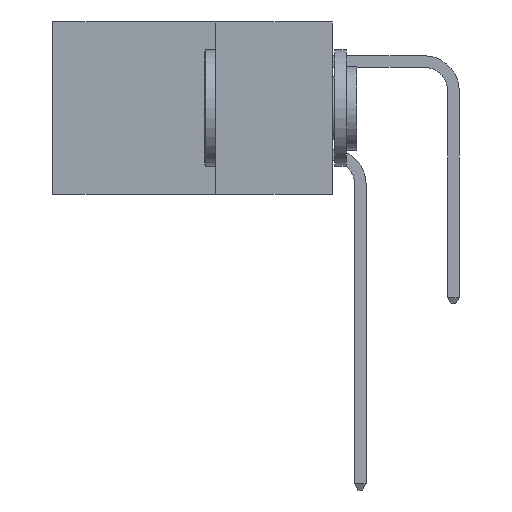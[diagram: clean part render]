
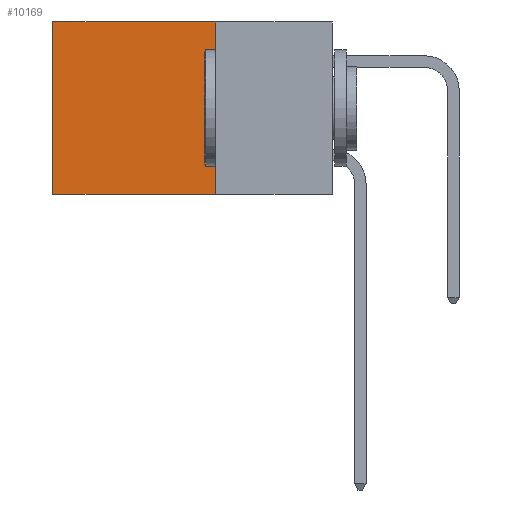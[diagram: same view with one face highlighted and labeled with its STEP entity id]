
A CAD part, left-side view. The second image highlights one B-rep face of the part: STEP entity #10169.
In plain terms, the highlighted planar face has unit normal (-1, 0, 0).
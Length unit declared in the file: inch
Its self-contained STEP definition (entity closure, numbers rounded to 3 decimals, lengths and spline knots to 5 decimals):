
#74 = LINE ( 'NONE', #7665, #5680 ) ;
#1587 = VECTOR ( 'NONE', #6917, 39.37008 ) ;
#1938 = VECTOR ( 'NONE', #3022, 39.37008 ) ;
#3015 = EDGE_LOOP ( 'NONE', ( #4439, #4606, #4668, #4705 ) ) ;
#3022 = DIRECTION ( 'NONE',  ( 0., 1., 0. ) ) ;
#3289 = VERTEX_POINT ( 'NONE', #12738 ) ;
#3512 = DIRECTION ( 'NONE',  ( 0., 0., -1. ) ) ;
#3734 = EDGE_CURVE ( 'NONE', #8182, #3289, #6736, .T. ) ;
#3924 = VECTOR ( 'NONE', #13265, 39.37008 ) ;
#4439 = ORIENTED_EDGE ( 'NONE', *, *, #6922, .T. ) ;
#4606 = ORIENTED_EDGE ( 'NONE', *, *, #10171, .F. ) ;
#4668 = ORIENTED_EDGE ( 'NONE', *, *, #6403, .F. ) ;
#4705 = ORIENTED_EDGE ( 'NONE', *, *, #3734, .T. ) ;
#5125 = PLANE ( 'NONE',  #8389 ) ;
#5680 = VECTOR ( 'NONE', #3512, 39.37008 ) ;
#5880 = CARTESIAN_POINT ( 'NONE',  ( 0.2615, 0.25, -0.37 ) ) ;
#6054 = CARTESIAN_POINT ( 'NONE',  ( 0.2615, 0.25, -0.37 ) ) ;
#6205 = CARTESIAN_POINT ( 'NONE',  ( 0.2615, 0.25, -0.37 ) ) ;
#6403 = EDGE_CURVE ( 'NONE', #8182, #12089, #6703, .T. ) ;
#6703 = LINE ( 'NONE', #5880, #1587 ) ;
#6736 = LINE ( 'NONE', #12322, #3924 ) ;
#6917 = DIRECTION ( 'NONE',  ( 0., 0., -1. ) ) ;
#6922 = EDGE_CURVE ( 'NONE', #3289, #6930, #74, .T. ) ;
#6930 = VERTEX_POINT ( 'NONE', #7709 ) ;
#7215 = DIRECTION ( 'NONE',  ( 0., 0., -1. ) ) ;
#7260 = CARTESIAN_POINT ( 'NONE',  ( 0.2615, 0.25, 0. ) ) ;
#7665 = CARTESIAN_POINT ( 'NONE',  ( 0.2615, 0.6, -0.37 ) ) ;
#7709 = CARTESIAN_POINT ( 'NONE',  ( 0.2615, 0.6, -0.37 ) ) ;
#8182 = VERTEX_POINT ( 'NONE', #7260 ) ;
#8389 = AXIS2_PLACEMENT_3D ( 'NONE', #6205, #13159, #7215 ) ;
#9312 = CARTESIAN_POINT ( 'NONE',  ( 0.2615, 0.25, -0.37 ) ) ;
#10169 = ADVANCED_FACE ( 'NONE', ( #12628 ), #5125, .F. ) ;
#10171 = EDGE_CURVE ( 'NONE', #12089, #6930, #13202, .T. ) ;
#12089 = VERTEX_POINT ( 'NONE', #6054 ) ;
#12322 = CARTESIAN_POINT ( 'NONE',  ( 0.2615, 0.25, 0. ) ) ;
#12628 = FACE_OUTER_BOUND ( 'NONE', #3015, .T. ) ;
#12738 = CARTESIAN_POINT ( 'NONE',  ( 0.2615, 0.6, 0. ) ) ;
#13159 = DIRECTION ( 'NONE',  ( 1., 0., 0. ) ) ;
#13202 = LINE ( 'NONE', #9312, #1938 ) ;
#13265 = DIRECTION ( 'NONE',  ( 0., 1., 0. ) ) ;
